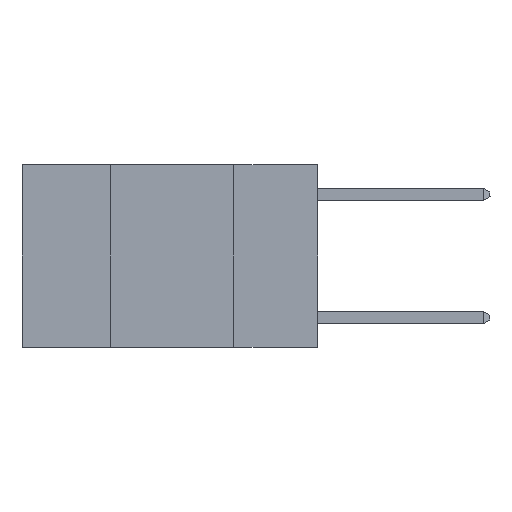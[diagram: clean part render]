
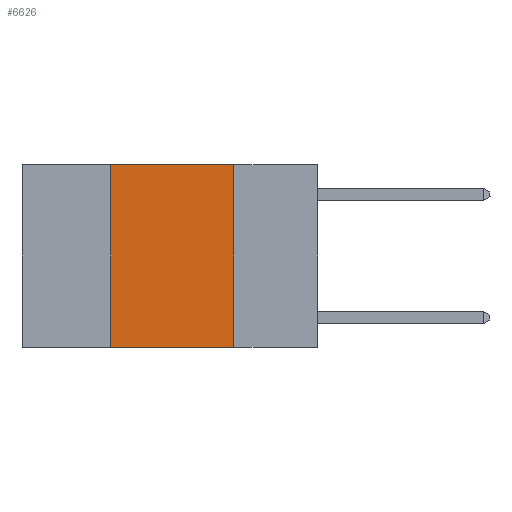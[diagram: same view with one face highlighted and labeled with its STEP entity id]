
A CAD part, left-side view. The second image highlights one B-rep face of the part: STEP entity #6626.
In plain terms, the highlighted planar face has unit normal (-1, 0, 0).
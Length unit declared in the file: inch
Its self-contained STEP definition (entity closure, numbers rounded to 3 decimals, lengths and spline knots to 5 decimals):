
#275 = DIRECTION ( 'NONE',  ( 0., -1., 0. ) ) ;
#338 = VECTOR ( 'NONE', #275, 39.37008 ) ;
#594 = CARTESIAN_POINT ( 'NONE',  ( 0., 0.6, -0.37 ) ) ;
#744 = CARTESIAN_POINT ( 'NONE',  ( 0., 0.6, 0. ) ) ;
#1781 = VECTOR ( 'NONE', #7224, 39.37008 ) ;
#1962 = CARTESIAN_POINT ( 'NONE',  ( 0., 0.42, 0. ) ) ;
#2264 = LINE ( 'NONE', #8481, #8628 ) ;
#3451 = VECTOR ( 'NONE', #4981, 39.37008 ) ;
#4096 = FACE_OUTER_BOUND ( 'NONE', #7605, .T. ) ;
#4313 = PLANE ( 'NONE',  #6761 ) ;
#4772 = VERTEX_POINT ( 'NONE', #1962 ) ;
#4797 = ORIENTED_EDGE ( 'NONE', *, *, #9269, .F. ) ;
#4981 = DIRECTION ( 'NONE',  ( 0., -1., 0. ) ) ;
#5313 = VERTEX_POINT ( 'NONE', #12924 ) ;
#5905 = EDGE_CURVE ( 'NONE', #4772, #12058, #8753, .T. ) ;
#6147 = ORIENTED_EDGE ( 'NONE', *, *, #5905, .F. ) ;
#6626 = ADVANCED_FACE ( 'NONE', ( #4096 ), #4313, .F. ) ;
#6761 = AXIS2_PLACEMENT_3D ( 'NONE', #744, #9120, #13741 ) ;
#7224 = DIRECTION ( 'NONE',  ( 0., 0., -1. ) ) ;
#7295 = VERTEX_POINT ( 'NONE', #10574 ) ;
#7605 = EDGE_LOOP ( 'NONE', ( #4797, #6147, #11507, #13964 ) ) ;
#8481 = CARTESIAN_POINT ( 'NONE',  ( 0., 0.42, 0. ) ) ;
#8628 = VECTOR ( 'NONE', #9512, 39.37008 ) ;
#8726 = CARTESIAN_POINT ( 'NONE',  ( 0., 0.17, 0. ) ) ;
#8753 = LINE ( 'NONE', #9927, #3451 ) ;
#9120 = DIRECTION ( 'NONE',  ( 1., 0., 0. ) ) ;
#9269 = EDGE_CURVE ( 'NONE', #12058, #5313, #14605, .T. ) ;
#9512 = DIRECTION ( 'NONE',  ( 0., 0., 1. ) ) ;
#9927 = CARTESIAN_POINT ( 'NONE',  ( 0., 0.6, 0. ) ) ;
#10574 = CARTESIAN_POINT ( 'NONE',  ( 0., 0.42, -0.37 ) ) ;
#11081 = LINE ( 'NONE', #594, #338 ) ;
#11507 = ORIENTED_EDGE ( 'NONE', *, *, #13025, .F. ) ;
#11892 = CARTESIAN_POINT ( 'NONE',  ( 0., 0.17, 0. ) ) ;
#12058 = VERTEX_POINT ( 'NONE', #11892 ) ;
#12924 = CARTESIAN_POINT ( 'NONE',  ( 0., 0.17, -0.37 ) ) ;
#13025 = EDGE_CURVE ( 'NONE', #7295, #4772, #2264, .T. ) ;
#13741 = DIRECTION ( 'NONE',  ( 0., 0., -1. ) ) ;
#13964 = ORIENTED_EDGE ( 'NONE', *, *, #14777, .T. ) ;
#14605 = LINE ( 'NONE', #8726, #1781 ) ;
#14777 = EDGE_CURVE ( 'NONE', #7295, #5313, #11081, .T. ) ;
